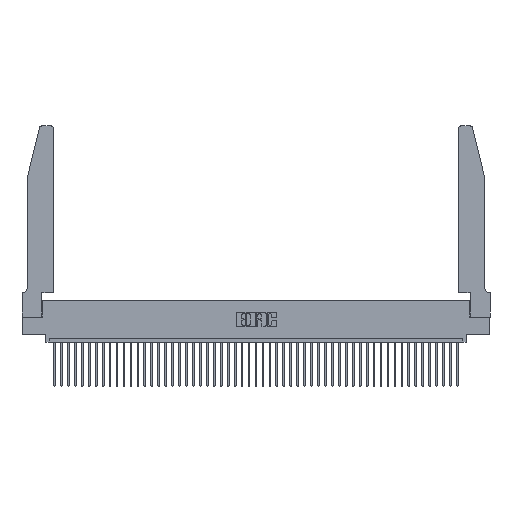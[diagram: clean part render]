
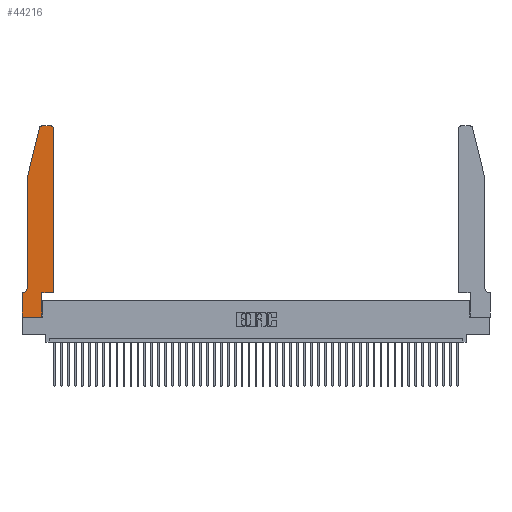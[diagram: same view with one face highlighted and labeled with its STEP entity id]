
A CAD part, top view. The second image highlights one B-rep face of the part: STEP entity #44216.
In plain terms, the highlighted planar face has unit normal (0, 0, 1).
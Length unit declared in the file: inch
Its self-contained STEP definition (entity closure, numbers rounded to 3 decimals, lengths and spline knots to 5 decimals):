
#428 = ORIENTED_EDGE ( 'NONE', *, *, #2514, .T. ) ;
#506 = DIRECTION ( 'NONE',  ( 1., 0., 0. ) ) ;
#1254 = EDGE_CURVE ( 'NONE', #14738, #10739, #28300, .T. ) ;
#1729 = EDGE_CURVE ( 'NONE', #38214, #36576, #34526, .T. ) ;
#2083 = EDGE_CURVE ( 'NONE', #5010, #14738, #12086, .T. ) ;
#2514 = EDGE_CURVE ( 'NONE', #18087, #20863, #12576, .T. ) ;
#3253 = VECTOR ( 'NONE', #46598, 39.37008 ) ;
#4845 = CARTESIAN_POINT ( 'NONE',  ( 0., 0.35, 0.37 ) ) ;
#4892 = CARTESIAN_POINT ( 'NONE',  ( 0.0755, 2., 0.37 ) ) ;
#5010 = VERTEX_POINT ( 'NONE', #18694 ) ;
#5101 = ORIENTED_EDGE ( 'NONE', *, *, #7458, .T. ) ;
#5848 = DIRECTION ( 'NONE',  ( 0., 0., 1. ) ) ;
#6588 = CARTESIAN_POINT ( 'NONE',  ( 0., 0.35, 0.37 ) ) ;
#7328 = CARTESIAN_POINT ( 'NONE',  ( 0.4505, 2.72, 0.37 ) ) ;
#7458 = EDGE_CURVE ( 'NONE', #36576, #11931, #15563, .T. ) ;
#7623 = DIRECTION ( 'NONE',  ( -1., 0., 0. ) ) ;
#8502 = EDGE_CURVE ( 'NONE', #36383, #38529, #22765, .T. ) ;
#8510 = VECTOR ( 'NONE', #32062, 39.37008 ) ;
#8689 = ORIENTED_EDGE ( 'NONE', *, *, #1254, .T. ) ;
#9786 = CARTESIAN_POINT ( 'NONE',  ( 0., 0., 0.37 ) ) ;
#10102 = VERTEX_POINT ( 'NONE', #14879 ) ;
#10462 = EDGE_CURVE ( 'NONE', #38529, #10102, #23712, .T. ) ;
#10739 = VERTEX_POINT ( 'NONE', #14843 ) ;
#10986 = CARTESIAN_POINT ( 'NONE',  ( 0.0055, 0.42, 0.37 ) ) ;
#11931 = VERTEX_POINT ( 'NONE', #36659 ) ;
#11988 = ORIENTED_EDGE ( 'NONE', *, *, #13551, .T. ) ;
#12086 = LINE ( 'NONE', #42594, #39957 ) ;
#12346 = DIRECTION ( 'NONE',  ( -0.239, -0.971, 0. ) ) ;
#12576 = LINE ( 'NONE', #18754, #36506 ) ;
#13119 = DIRECTION ( 'NONE',  ( 0., -1., 0. ) ) ;
#13551 = EDGE_CURVE ( 'NONE', #27167, #36383, #23353, .T. ) ;
#13604 = AXIS2_PLACEMENT_3D ( 'NONE', #10986, #43836, #7623 ) ;
#13798 = FACE_OUTER_BOUND ( 'NONE', #15728, .T. ) ;
#14655 = ORIENTED_EDGE ( 'NONE', *, *, #10462, .T. ) ;
#14738 = VERTEX_POINT ( 'NONE', #6588 ) ;
#14843 = CARTESIAN_POINT ( 'NONE',  ( 0., 0., 0.37 ) ) ;
#14879 = CARTESIAN_POINT ( 'NONE',  ( 0.284, 2.75, 0.37 ) ) ;
#15563 = LINE ( 'NONE', #34899, #32674 ) ;
#15628 = EDGE_CURVE ( 'NONE', #20863, #27167, #40913, .T. ) ;
#15728 = EDGE_LOOP ( 'NONE', ( #14655, #19019, #38530, #5101, #37912, #41158, #8689, #17849, #428, #24192, #11988, #30960 ) ) ;
#17412 = EDGE_CURVE ( 'NONE', #10102, #38214, #47011, .T. ) ;
#17849 = ORIENTED_EDGE ( 'NONE', *, *, #33147, .T. ) ;
#18087 = VERTEX_POINT ( 'NONE', #28418 ) ;
#18694 = CARTESIAN_POINT ( 'NONE',  ( 0.0055, 0.35, 0.37 ) ) ;
#18754 = CARTESIAN_POINT ( 'NONE',  ( 0.2865, 0.35, 0.37 ) ) ;
#18796 = VECTOR ( 'NONE', #27832, 39.37008 ) ;
#19019 = ORIENTED_EDGE ( 'NONE', *, *, #17412, .T. ) ;
#19943 = DIRECTION ( 'NONE',  ( 0., 0., 1. ) ) ;
#20863 = VERTEX_POINT ( 'NONE', #39135 ) ;
#22234 = CARTESIAN_POINT ( 'NONE',  ( 0.4505, 0.35, 0.37 ) ) ;
#22765 = CIRCLE ( 'NONE', #26964, 0.03 ) ;
#23353 = LINE ( 'NONE', #34621, #18796 ) ;
#23471 = DIRECTION ( 'NONE',  ( 1., 0., 0. ) ) ;
#23607 = CIRCLE ( 'NONE', #13604, 0.07 ) ;
#23712 = LINE ( 'NONE', #43153, #3253 ) ;
#23962 = CARTESIAN_POINT ( 'NONE',  ( 0.284, 2.72, 0.37 ) ) ;
#24192 = ORIENTED_EDGE ( 'NONE', *, *, #15628, .T. ) ;
#24785 = DIRECTION ( 'NONE',  ( 1., 0., 0. ) ) ;
#25921 = DIRECTION ( 'NONE',  ( 0., 1., 0. ) ) ;
#26964 = AXIS2_PLACEMENT_3D ( 'NONE', #30484, #34124, #23471 ) ;
#27167 = VERTEX_POINT ( 'NONE', #22234 ) ;
#27832 = DIRECTION ( 'NONE',  ( 0., 1., 0. ) ) ;
#28072 = DIRECTION ( 'NONE',  ( 0., -1., 0. ) ) ;
#28300 = LINE ( 'NONE', #9786, #41316 ) ;
#28418 = CARTESIAN_POINT ( 'NONE',  ( 0.2865, 0., 0.37 ) ) ;
#30045 = CARTESIAN_POINT ( 'NONE',  ( 0.0755, 2., 0.37 ) ) ;
#30484 = CARTESIAN_POINT ( 'NONE',  ( 0.4205, 2.72, 0.37 ) ) ;
#30960 = ORIENTED_EDGE ( 'NONE', *, *, #8502, .T. ) ;
#32062 = DIRECTION ( 'NONE',  ( 1., 0., 0. ) ) ;
#32384 = CARTESIAN_POINT ( 'NONE',  ( 0., 0., 0.37 ) ) ;
#32674 = VECTOR ( 'NONE', #13119, 39.37008 ) ;
#33087 = CARTESIAN_POINT ( 'NONE',  ( 0.4505, 0.35, 0.37 ) ) ;
#33147 = EDGE_CURVE ( 'NONE', #10739, #18087, #39788, .T. ) ;
#33229 = AXIS2_PLACEMENT_3D ( 'NONE', #4845, #19943, #41077 ) ;
#34124 = DIRECTION ( 'NONE',  ( 0., 0., 1. ) ) ;
#34526 = LINE ( 'NONE', #4892, #39598 ) ;
#34621 = CARTESIAN_POINT ( 'NONE',  ( 0.4505, 0.35, 0.37 ) ) ;
#34675 = VECTOR ( 'NONE', #506, 39.37008 ) ;
#34899 = CARTESIAN_POINT ( 'NONE',  ( 0.0755, 2., 0.37 ) ) ;
#35591 = EDGE_CURVE ( 'NONE', #11931, #5010, #23607, .T. ) ;
#36357 = CARTESIAN_POINT ( 'NONE',  ( 0.4205, 2.75, 0.37 ) ) ;
#36383 = VERTEX_POINT ( 'NONE', #7328 ) ;
#36506 = VECTOR ( 'NONE', #25921, 39.37008 ) ;
#36576 = VERTEX_POINT ( 'NONE', #30045 ) ;
#36659 = CARTESIAN_POINT ( 'NONE',  ( 0.0755, 0.42, 0.37 ) ) ;
#37912 = ORIENTED_EDGE ( 'NONE', *, *, #35591, .T. ) ;
#38214 = VERTEX_POINT ( 'NONE', #41603 ) ;
#38529 = VERTEX_POINT ( 'NONE', #36357 ) ;
#38530 = ORIENTED_EDGE ( 'NONE', *, *, #1729, .T. ) ;
#38623 = DIRECTION ( 'NONE',  ( -1., 0., 0. ) ) ;
#39135 = CARTESIAN_POINT ( 'NONE',  ( 0.2865, 0.35, 0.37 ) ) ;
#39598 = VECTOR ( 'NONE', #12346, 39.37008 ) ;
#39788 = LINE ( 'NONE', #32384, #8510 ) ;
#39957 = VECTOR ( 'NONE', #38623, 39.37008 ) ;
#40913 = LINE ( 'NONE', #33087, #34675 ) ;
#41077 = DIRECTION ( 'NONE',  ( 1., 0., 0. ) ) ;
#41158 = ORIENTED_EDGE ( 'NONE', *, *, #2083, .T. ) ;
#41228 = PLANE ( 'NONE',  #33229 ) ;
#41316 = VECTOR ( 'NONE', #28072, 39.37008 ) ;
#41603 = CARTESIAN_POINT ( 'NONE',  ( 0.25487, 2.72718, 0.37 ) ) ;
#41758 = AXIS2_PLACEMENT_3D ( 'NONE', #23962, #5848, #24785 ) ;
#42594 = CARTESIAN_POINT ( 'NONE',  ( 0.0755, 0.35, 0.37 ) ) ;
#43153 = CARTESIAN_POINT ( 'NONE',  ( 0.2605, 2.75, 0.37 ) ) ;
#43836 = DIRECTION ( 'NONE',  ( 0., 0., -1. ) ) ;
#44216 = ADVANCED_FACE ( 'NONE', ( #13798 ), #41228, .T. ) ;
#46598 = DIRECTION ( 'NONE',  ( -1., 0., 0. ) ) ;
#47011 = CIRCLE ( 'NONE', #41758, 0.03 ) ;
